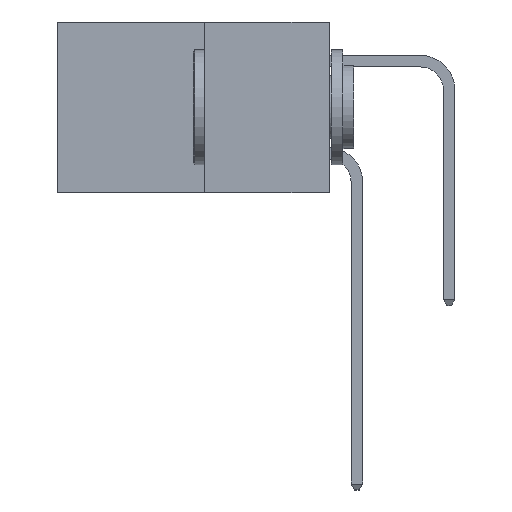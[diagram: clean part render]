
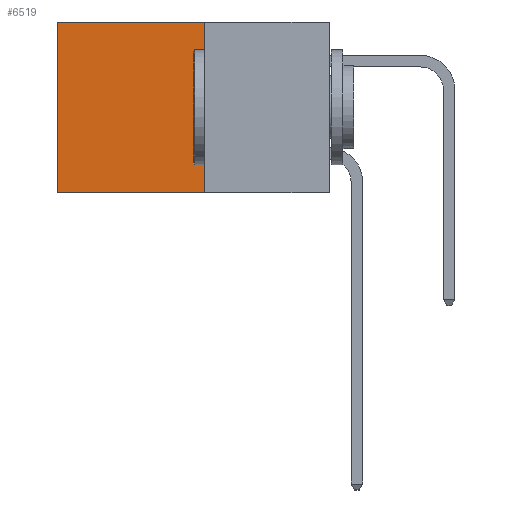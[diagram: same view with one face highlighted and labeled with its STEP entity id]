
A CAD part, left-side view. The second image highlights one B-rep face of the part: STEP entity #6519.
In plain terms, the highlighted planar face has unit normal (-1, 0, 0).
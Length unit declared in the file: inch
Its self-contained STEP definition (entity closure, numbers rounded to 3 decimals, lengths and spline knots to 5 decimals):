
#475 = ORIENTED_EDGE ( 'NONE', *, *, #11495, .T. ) ;
#1512 = VERTEX_POINT ( 'NONE', #6480 ) ;
#2016 = ORIENTED_EDGE ( 'NONE', *, *, #12501, .F. ) ;
#3111 = VECTOR ( 'NONE', #11983, 39.37008 ) ;
#3225 = DIRECTION ( 'NONE',  ( 0., 0., -1. ) ) ;
#3348 = AXIS2_PLACEMENT_3D ( 'NONE', #7632, #7619, #7503 ) ;
#3887 = VERTEX_POINT ( 'NONE', #10997 ) ;
#4220 = CARTESIAN_POINT ( 'NONE',  ( 0.277, 0.27, -0.37 ) ) ;
#4939 = LINE ( 'NONE', #4220, #10339 ) ;
#5193 = ORIENTED_EDGE ( 'NONE', *, *, #5246, .T. ) ;
#5246 = EDGE_CURVE ( 'NONE', #5397, #1512, #9090, .T. ) ;
#5298 = FACE_OUTER_BOUND ( 'NONE', #12818, .T. ) ;
#5397 = VERTEX_POINT ( 'NONE', #12588 ) ;
#5716 = CARTESIAN_POINT ( 'NONE',  ( 0.277, 0.59, -0.37 ) ) ;
#6292 = VECTOR ( 'NONE', #10098, 39.37008 ) ;
#6480 = CARTESIAN_POINT ( 'NONE',  ( 0.277, 0.59, 0. ) ) ;
#6519 = ADVANCED_FACE ( 'NONE', ( #5298 ), #7693, .F. ) ;
#6908 = CARTESIAN_POINT ( 'NONE',  ( 0.277, 0.27, -0.37 ) ) ;
#7503 = DIRECTION ( 'NONE',  ( 0., 0., -1. ) ) ;
#7619 = DIRECTION ( 'NONE',  ( 1., 0., 0. ) ) ;
#7632 = CARTESIAN_POINT ( 'NONE',  ( 0.277, 0.27, -0.37 ) ) ;
#7693 = PLANE ( 'NONE',  #3348 ) ;
#8135 = EDGE_CURVE ( 'NONE', #8820, #3887, #12232, .T. ) ;
#8820 = VERTEX_POINT ( 'NONE', #6908 ) ;
#9090 = LINE ( 'NONE', #12011, #3111 ) ;
#9228 = LINE ( 'NONE', #5716, #6292 ) ;
#9540 = VECTOR ( 'NONE', #10790, 39.37008 ) ;
#10098 = DIRECTION ( 'NONE',  ( 0., 0., -1. ) ) ;
#10339 = VECTOR ( 'NONE', #3225, 39.37008 ) ;
#10790 = DIRECTION ( 'NONE',  ( 0., 1., 0. ) ) ;
#10844 = CARTESIAN_POINT ( 'NONE',  ( 0.277, 0.27, -0.37 ) ) ;
#10997 = CARTESIAN_POINT ( 'NONE',  ( 0.277, 0.59, -0.37 ) ) ;
#11495 = EDGE_CURVE ( 'NONE', #1512, #3887, #9228, .T. ) ;
#11983 = DIRECTION ( 'NONE',  ( 0., 1., 0. ) ) ;
#12011 = CARTESIAN_POINT ( 'NONE',  ( 0.277, 0.27, 0. ) ) ;
#12232 = LINE ( 'NONE', #10844, #9540 ) ;
#12401 = ORIENTED_EDGE ( 'NONE', *, *, #8135, .F. ) ;
#12501 = EDGE_CURVE ( 'NONE', #5397, #8820, #4939, .T. ) ;
#12588 = CARTESIAN_POINT ( 'NONE',  ( 0.277, 0.27, 0. ) ) ;
#12818 = EDGE_LOOP ( 'NONE', ( #475, #12401, #2016, #5193 ) ) ;
